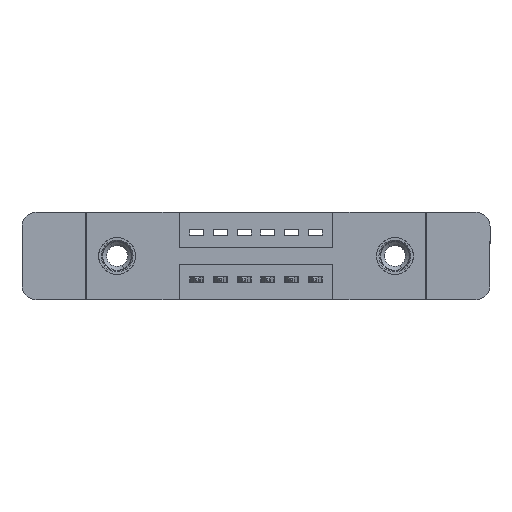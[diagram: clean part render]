
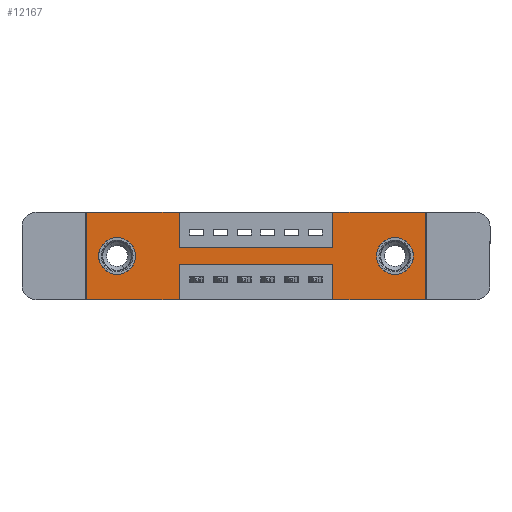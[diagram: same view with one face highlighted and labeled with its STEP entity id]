
A CAD part, front view. The second image highlights one B-rep face of the part: STEP entity #12167.
In plain terms, the highlighted planar face has unit normal (0, -1, 0).
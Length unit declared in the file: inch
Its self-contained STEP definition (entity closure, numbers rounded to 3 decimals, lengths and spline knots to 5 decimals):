
#275 = CARTESIAN_POINT ( 'NONE',  ( 0.13, 0., -0.107 ) ) ;
#397 = VECTOR ( 'NONE', #13384, 39.37008 ) ;
#573 = EDGE_CURVE ( 'NONE', #8426, #3622, #6880, .T. ) ;
#618 = DIRECTION ( 'NONE',  ( -1., 0., 0. ) ) ;
#713 = CARTESIAN_POINT ( 'NONE',  ( 0., 0., 0. ) ) ;
#794 = CARTESIAN_POINT ( 'NONE',  ( 0.13, 0., -0.263 ) ) ;
#932 = CARTESIAN_POINT ( 'NONE',  ( 0.3925, 0., -0.22 ) ) ;
#1024 = ORIENTED_EDGE ( 'NONE', *, *, #4578, .F. ) ;
#1155 = VECTOR ( 'NONE', #7691, 39.37008 ) ;
#1164 = DIRECTION ( 'NONE',  ( 0., 0., -1. ) ) ;
#1240 = CARTESIAN_POINT ( 'NONE',  ( 1.305, 0., -0.185 ) ) ;
#1241 = EDGE_CURVE ( 'NONE', #13135, #13446, #1715, .T. ) ;
#1245 = ORIENTED_EDGE ( 'NONE', *, *, #9402, .T. ) ;
#1255 = CARTESIAN_POINT ( 'NONE',  ( 1.0425, 0., -0.22 ) ) ;
#1256 = DIRECTION ( 'NONE',  ( 0., 1., 0. ) ) ;
#1454 = LINE ( 'NONE', #11410, #3404 ) ;
#1644 = CARTESIAN_POINT ( 'NONE',  ( 0., 0., -0.37 ) ) ;
#1715 = CIRCLE ( 'NONE', #1923, 0.078 ) ;
#1740 = VERTEX_POINT ( 'NONE', #7809 ) ;
#1839 = CARTESIAN_POINT ( 'NONE',  ( 1.435, 0., 0. ) ) ;
#1885 = ORIENTED_EDGE ( 'NONE', *, *, #11880, .F. ) ;
#1923 = AXIS2_PLACEMENT_3D ( 'NONE', #8143, #1256, #6882 ) ;
#2161 = ORIENTED_EDGE ( 'NONE', *, *, #1241, .T. ) ;
#2197 = EDGE_CURVE ( 'NONE', #3622, #12407, #9437, .T. ) ;
#2282 = CARTESIAN_POINT ( 'NONE',  ( 1.305, 0., -0.185 ) ) ;
#2368 = DIRECTION ( 'NONE',  ( 0., 0., -1. ) ) ;
#2467 = DIRECTION ( 'NONE',  ( -1., 0., 0. ) ) ;
#2529 = DIRECTION ( 'NONE',  ( 0., 0., 1. ) ) ;
#2746 = DIRECTION ( 'NONE',  ( 0., -1., 0. ) ) ;
#2892 = ORIENTED_EDGE ( 'NONE', *, *, #13401, .F. ) ;
#3010 = CARTESIAN_POINT ( 'NONE',  ( 0.3925, 0., -0.15 ) ) ;
#3070 = DIRECTION ( 'NONE',  ( 0., 0., -1. ) ) ;
#3170 = CARTESIAN_POINT ( 'NONE',  ( 0.3925, 0., -0.37 ) ) ;
#3220 = CARTESIAN_POINT ( 'NONE',  ( 0.3925, 0., -0.15 ) ) ;
#3337 = VECTOR ( 'NONE', #2529, 39.37008 ) ;
#3371 = CIRCLE ( 'NONE', #9895, 0.078 ) ;
#3404 = VECTOR ( 'NONE', #2467, 39.37008 ) ;
#3407 = ORIENTED_EDGE ( 'NONE', *, *, #573, .F. ) ;
#3467 = CARTESIAN_POINT ( 'NONE',  ( 0., 0., 0. ) ) ;
#3622 = VERTEX_POINT ( 'NONE', #9435 ) ;
#3849 = VECTOR ( 'NONE', #11868, 39.37008 ) ;
#3908 = FACE_BOUND ( 'NONE', #6477, .T. ) ;
#4088 = VECTOR ( 'NONE', #12776, 39.37008 ) ;
#4107 = EDGE_CURVE ( 'NONE', #13301, #13536, #9762, .T. ) ;
#4264 = LINE ( 'NONE', #3010, #12852 ) ;
#4472 = FACE_OUTER_BOUND ( 'NONE', #9186, .T. ) ;
#4578 = EDGE_CURVE ( 'NONE', #14295, #13301, #7401, .T. ) ;
#4710 = DIRECTION ( 'NONE',  ( 1., 0., 0. ) ) ;
#4925 = EDGE_CURVE ( 'NONE', #13536, #12950, #12480, .T. ) ;
#5342 = FACE_BOUND ( 'NONE', #10134, .T. ) ;
#5872 = AXIS2_PLACEMENT_3D ( 'NONE', #1240, #6866, #2368 ) ;
#5950 = VECTOR ( 'NONE', #4710, 39.37008 ) ;
#6065 = ORIENTED_EDGE ( 'NONE', *, *, #2197, .F. ) ;
#6110 = ORIENTED_EDGE ( 'NONE', *, *, #7045, .F. ) ;
#6118 = DIRECTION ( 'NONE',  ( 0., 0., -1. ) ) ;
#6477 = EDGE_LOOP ( 'NONE', ( #2161, #1245 ) ) ;
#6669 = CARTESIAN_POINT ( 'NONE',  ( 0.3925, 0., 0. ) ) ;
#6685 = CARTESIAN_POINT ( 'NONE',  ( 1.0425, 0., -0.37 ) ) ;
#6829 = VECTOR ( 'NONE', #3070, 39.37008 ) ;
#6866 = DIRECTION ( 'NONE',  ( 0., 1., 0. ) ) ;
#6880 = LINE ( 'NONE', #713, #7226 ) ;
#6882 = DIRECTION ( 'NONE',  ( 0., 0., 1. ) ) ;
#7002 = CARTESIAN_POINT ( 'NONE',  ( 0.3925, 0., 0. ) ) ;
#7045 = EDGE_CURVE ( 'NONE', #12357, #8426, #7717, .T. ) ;
#7226 = VECTOR ( 'NONE', #14130, 39.37008 ) ;
#7251 = CARTESIAN_POINT ( 'NONE',  ( 0.13, 0., -0.185 ) ) ;
#7335 = VERTEX_POINT ( 'NONE', #11106 ) ;
#7345 = CARTESIAN_POINT ( 'NONE',  ( 0., 0., -0.37 ) ) ;
#7401 = LINE ( 'NONE', #1839, #3849 ) ;
#7413 = EDGE_CURVE ( 'NONE', #9731, #12357, #12431, .T. ) ;
#7420 = CIRCLE ( 'NONE', #5872, 0.078 ) ;
#7459 = ORIENTED_EDGE ( 'NONE', *, *, #13684, .T. ) ;
#7614 = AXIS2_PLACEMENT_3D ( 'NONE', #7345, #2746, #6118 ) ;
#7663 = VECTOR ( 'NONE', #13680, 39.37008 ) ;
#7691 = DIRECTION ( 'NONE',  ( -1., 0., 0. ) ) ;
#7717 = LINE ( 'NONE', #1644, #12260 ) ;
#7809 = CARTESIAN_POINT ( 'NONE',  ( 1.0425, 0., 0. ) ) ;
#7846 = CARTESIAN_POINT ( 'NONE',  ( 0.3925, 0., -0.37 ) ) ;
#8143 = CARTESIAN_POINT ( 'NONE',  ( 0.13, 0., -0.185 ) ) ;
#8181 = CARTESIAN_POINT ( 'NONE',  ( 1.435, 0., 0. ) ) ;
#8331 = LINE ( 'NONE', #12542, #7663 ) ;
#8426 = VERTEX_POINT ( 'NONE', #13173 ) ;
#8557 = VERTEX_POINT ( 'NONE', #10182 ) ;
#8851 = LINE ( 'NONE', #7002, #4088 ) ;
#9052 = VERTEX_POINT ( 'NONE', #3220 ) ;
#9177 = EDGE_CURVE ( 'NONE', #7335, #1740, #8331, .T. ) ;
#9186 = EDGE_LOOP ( 'NONE', ( #11343, #1885, #9633, #13635, #1024, #14094, #12110, #2892, #13867, #6065, #3407, #6110 ) ) ;
#9402 = EDGE_CURVE ( 'NONE', #13446, #13135, #13598, .T. ) ;
#9435 = CARTESIAN_POINT ( 'NONE',  ( 0., 0., 0. ) ) ;
#9437 = LINE ( 'NONE', #3467, #5950 ) ;
#9532 = DIRECTION ( 'NONE',  ( 0., 1., 0. ) ) ;
#9633 = ORIENTED_EDGE ( 'NONE', *, *, #4925, .F. ) ;
#9731 = VERTEX_POINT ( 'NONE', #932 ) ;
#9737 = EDGE_CURVE ( 'NONE', #1740, #14295, #12358, .T. ) ;
#9762 = LINE ( 'NONE', #14381, #1155 ) ;
#9828 = AXIS2_PLACEMENT_3D ( 'NONE', #7251, #9532, #10656 ) ;
#9895 = AXIS2_PLACEMENT_3D ( 'NONE', #2282, #11919, #1164 ) ;
#10134 = EDGE_LOOP ( 'NONE', ( #7459, #13292 ) ) ;
#10182 = CARTESIAN_POINT ( 'NONE',  ( 1.305, 0., -0.107 ) ) ;
#10316 = VERTEX_POINT ( 'NONE', #12026 ) ;
#10656 = DIRECTION ( 'NONE',  ( 0., 0., 1. ) ) ;
#11106 = CARTESIAN_POINT ( 'NONE',  ( 1.0425, 0., -0.15 ) ) ;
#11343 = ORIENTED_EDGE ( 'NONE', *, *, #7413, .F. ) ;
#11410 = CARTESIAN_POINT ( 'NONE',  ( 0.3925, 0., -0.22 ) ) ;
#11868 = DIRECTION ( 'NONE',  ( 0., 0., -1. ) ) ;
#11880 = EDGE_CURVE ( 'NONE', #12950, #9731, #1454, .T. ) ;
#11919 = DIRECTION ( 'NONE',  ( 0., 1., 0. ) ) ;
#11997 = EDGE_CURVE ( 'NONE', #12407, #9052, #8851, .T. ) ;
#12026 = CARTESIAN_POINT ( 'NONE',  ( 1.305, 0., -0.263 ) ) ;
#12110 = ORIENTED_EDGE ( 'NONE', *, *, #9177, .F. ) ;
#12167 = ADVANCED_FACE ( 'NONE', ( #5342, #3908, #4472 ), #12822, .T. ) ;
#12197 = CARTESIAN_POINT ( 'NONE',  ( 0., 0., 0. ) ) ;
#12260 = VECTOR ( 'NONE', #618, 39.37008 ) ;
#12357 = VERTEX_POINT ( 'NONE', #7846 ) ;
#12358 = LINE ( 'NONE', #12197, #397 ) ;
#12407 = VERTEX_POINT ( 'NONE', #6669 ) ;
#12431 = LINE ( 'NONE', #3170, #6829 ) ;
#12480 = LINE ( 'NONE', #12740, #3337 ) ;
#12542 = CARTESIAN_POINT ( 'NONE',  ( 1.0425, 0., 0. ) ) ;
#12740 = CARTESIAN_POINT ( 'NONE',  ( 1.0425, 0., -0.37 ) ) ;
#12776 = DIRECTION ( 'NONE',  ( 0., 0., -1. ) ) ;
#12822 = PLANE ( 'NONE',  #7614 ) ;
#12852 = VECTOR ( 'NONE', #14169, 39.37008 ) ;
#12950 = VERTEX_POINT ( 'NONE', #1255 ) ;
#13135 = VERTEX_POINT ( 'NONE', #275 ) ;
#13173 = CARTESIAN_POINT ( 'NONE',  ( 0., 0., -0.37 ) ) ;
#13292 = ORIENTED_EDGE ( 'NONE', *, *, #13703, .T. ) ;
#13301 = VERTEX_POINT ( 'NONE', #13920 ) ;
#13384 = DIRECTION ( 'NONE',  ( 1., 0., 0. ) ) ;
#13401 = EDGE_CURVE ( 'NONE', #9052, #7335, #4264, .T. ) ;
#13446 = VERTEX_POINT ( 'NONE', #794 ) ;
#13536 = VERTEX_POINT ( 'NONE', #6685 ) ;
#13598 = CIRCLE ( 'NONE', #9828, 0.078 ) ;
#13635 = ORIENTED_EDGE ( 'NONE', *, *, #4107, .F. ) ;
#13680 = DIRECTION ( 'NONE',  ( 0., 0., 1. ) ) ;
#13684 = EDGE_CURVE ( 'NONE', #8557, #10316, #7420, .T. ) ;
#13703 = EDGE_CURVE ( 'NONE', #10316, #8557, #3371, .T. ) ;
#13867 = ORIENTED_EDGE ( 'NONE', *, *, #11997, .F. ) ;
#13920 = CARTESIAN_POINT ( 'NONE',  ( 1.435, 0., -0.37 ) ) ;
#14094 = ORIENTED_EDGE ( 'NONE', *, *, #9737, .F. ) ;
#14130 = DIRECTION ( 'NONE',  ( 0., 0., 1. ) ) ;
#14169 = DIRECTION ( 'NONE',  ( 1., 0., 0. ) ) ;
#14295 = VERTEX_POINT ( 'NONE', #8181 ) ;
#14381 = CARTESIAN_POINT ( 'NONE',  ( 0., 0., -0.37 ) ) ;
